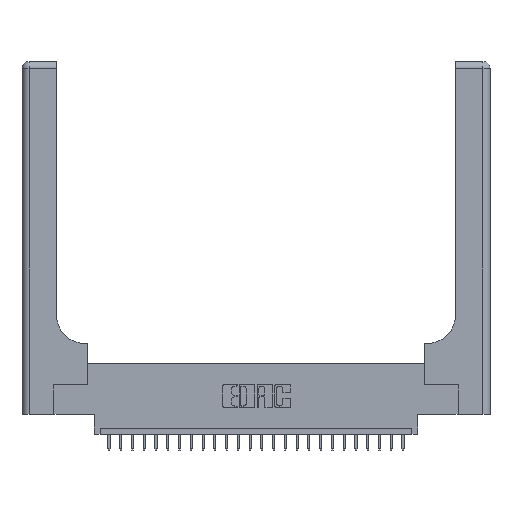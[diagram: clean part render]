
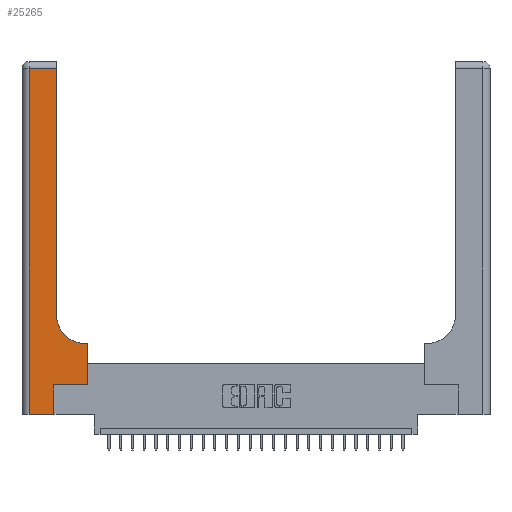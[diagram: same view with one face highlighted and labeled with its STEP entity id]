
A CAD part, top view. The second image highlights one B-rep face of the part: STEP entity #25265.
In plain terms, the highlighted planar face has unit normal (0, 0, 1).
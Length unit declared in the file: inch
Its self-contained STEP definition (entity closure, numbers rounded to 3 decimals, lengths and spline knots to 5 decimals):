
#173 = FACE_OUTER_BOUND ( 'NONE', #19217, .T. ) ;
#336 = EDGE_CURVE ( 'NONE', #24776, #21754, #4469, .T. ) ;
#856 = CARTESIAN_POINT ( 'NONE',  ( 0.2915, 3., 0.37 ) ) ;
#1157 = VERTEX_POINT ( 'NONE', #17591 ) ;
#1690 = VECTOR ( 'NONE', #5617, 39.37008 ) ;
#2215 = PLANE ( 'NONE',  #20758 ) ;
#3052 = VECTOR ( 'NONE', #19072, 39.37008 ) ;
#3142 = DIRECTION ( 'NONE',  ( 1., 0., 0. ) ) ;
#3426 = CIRCLE ( 'NONE', #19691, 0.25 ) ;
#4469 = LINE ( 'NONE', #856, #15046 ) ;
#4856 = CARTESIAN_POINT ( 'NONE',  ( 0.269, 0., 0.37 ) ) ;
#5480 = VECTOR ( 'NONE', #9628, 39.37008 ) ;
#5617 = DIRECTION ( 'NONE',  ( 1., 0., 0. ) ) ;
#5898 = ORIENTED_EDGE ( 'NONE', *, *, #18238, .T. ) ;
#6192 = CARTESIAN_POINT ( 'NONE',  ( 0.269, 0., 0.37 ) ) ;
#6291 = CARTESIAN_POINT ( 'NONE',  ( 0.2915, 2.94, 0.37 ) ) ;
#7305 = LINE ( 'NONE', #24150, #12107 ) ;
#7981 = DIRECTION ( 'NONE',  ( 1., 0., 0. ) ) ;
#8117 = CARTESIAN_POINT ( 'NONE',  ( 0.06, 2.94, 0.37 ) ) ;
#8766 = DIRECTION ( 'NONE',  ( 0., 1., 0. ) ) ;
#9373 = CARTESIAN_POINT ( 'NONE',  ( 0.06, 3., 0.37 ) ) ;
#9628 = DIRECTION ( 'NONE',  ( 0., -1., 0. ) ) ;
#10048 = CARTESIAN_POINT ( 'NONE',  ( 0.5415, 0.85, 0.37 ) ) ;
#10485 = VERTEX_POINT ( 'NONE', #26332 ) ;
#11897 = DIRECTION ( 'NONE',  ( -1., 0., 0. ) ) ;
#12107 = VECTOR ( 'NONE', #3142, 39.37008 ) ;
#12230 = LINE ( 'NONE', #6192, #26948 ) ;
#12709 = ORIENTED_EDGE ( 'NONE', *, *, #25765, .T. ) ;
#12770 = VERTEX_POINT ( 'NONE', #22653 ) ;
#12938 = ORIENTED_EDGE ( 'NONE', *, *, #22684, .T. ) ;
#13217 = VECTOR ( 'NONE', #22682, 39.37008 ) ;
#13233 = CARTESIAN_POINT ( 'NONE',  ( 0.5415, 0.6, 0.37 ) ) ;
#13918 = ORIENTED_EDGE ( 'NONE', *, *, #21764, .T. ) ;
#13954 = CARTESIAN_POINT ( 'NONE',  ( 0.2915, 0.6, 0.37 ) ) ;
#14596 = EDGE_CURVE ( 'NONE', #10485, #17119, #7305, .T. ) ;
#14833 = ORIENTED_EDGE ( 'NONE', *, *, #25785, .T. ) ;
#15046 = VECTOR ( 'NONE', #8766, 39.37008 ) ;
#16049 = LINE ( 'NONE', #24521, #1690 ) ;
#16080 = DIRECTION ( 'NONE',  ( 0., 0., -1. ) ) ;
#16294 = CARTESIAN_POINT ( 'NONE',  ( 0.269, 0.25, 0.37 ) ) ;
#16975 = DIRECTION ( 'NONE',  ( 0., 0., -1. ) ) ;
#17119 = VERTEX_POINT ( 'NONE', #4856 ) ;
#17133 = VERTEX_POINT ( 'NONE', #13233 ) ;
#17591 = CARTESIAN_POINT ( 'NONE',  ( 0.5585, 0.6, 0.37 ) ) ;
#17666 = VERTEX_POINT ( 'NONE', #16294 ) ;
#17807 = LINE ( 'NONE', #13954, #24451 ) ;
#18238 = EDGE_CURVE ( 'NONE', #17133, #24776, #3426, .T. ) ;
#18858 = ORIENTED_EDGE ( 'NONE', *, *, #336, .T. ) ;
#19072 = DIRECTION ( 'NONE',  ( 0., 1., 0. ) ) ;
#19217 = EDGE_LOOP ( 'NONE', ( #18858, #12938, #12709, #26934, #14833, #20153, #13918, #20929, #5898 ) ) ;
#19249 = VERTEX_POINT ( 'NONE', #8117 ) ;
#19691 = AXIS2_PLACEMENT_3D ( 'NONE', #10048, #16080, #7981 ) ;
#20153 = ORIENTED_EDGE ( 'NONE', *, *, #20202, .T. ) ;
#20202 = EDGE_CURVE ( 'NONE', #17666, #12770, #16049, .T. ) ;
#20460 = LINE ( 'NONE', #9373, #5480 ) ;
#20758 = AXIS2_PLACEMENT_3D ( 'NONE', #21221, #16975, #25290 ) ;
#20929 = ORIENTED_EDGE ( 'NONE', *, *, #26459, .T. ) ;
#21221 = CARTESIAN_POINT ( 'NONE',  ( 0., 3., 0.37 ) ) ;
#21754 = VERTEX_POINT ( 'NONE', #6291 ) ;
#21764 = EDGE_CURVE ( 'NONE', #12770, #1157, #25187, .T. ) ;
#22405 = CARTESIAN_POINT ( 'NONE',  ( 0.2915, 0.85, 0.37 ) ) ;
#22653 = CARTESIAN_POINT ( 'NONE',  ( 0.5585, 0.25, 0.37 ) ) ;
#22682 = DIRECTION ( 'NONE',  ( -1., 0., 0. ) ) ;
#22684 = EDGE_CURVE ( 'NONE', #21754, #19249, #24724, .T. ) ;
#22777 = DIRECTION ( 'NONE',  ( 0., 1., 0. ) ) ;
#23145 = CARTESIAN_POINT ( 'NONE',  ( 0.5585, 0.25, 0.37 ) ) ;
#24150 = CARTESIAN_POINT ( 'NONE',  ( 0., 0., 0.37 ) ) ;
#24451 = VECTOR ( 'NONE', #11897, 39.37008 ) ;
#24521 = CARTESIAN_POINT ( 'NONE',  ( 0.269, 0.25, 0.37 ) ) ;
#24724 = LINE ( 'NONE', #26382, #13217 ) ;
#24776 = VERTEX_POINT ( 'NONE', #22405 ) ;
#25187 = LINE ( 'NONE', #23145, #3052 ) ;
#25265 = ADVANCED_FACE ( 'NONE', ( #173 ), #2215, .F. ) ;
#25290 = DIRECTION ( 'NONE',  ( -1., 0., 0. ) ) ;
#25765 = EDGE_CURVE ( 'NONE', #19249, #10485, #20460, .T. ) ;
#25785 = EDGE_CURVE ( 'NONE', #17119, #17666, #12230, .T. ) ;
#26332 = CARTESIAN_POINT ( 'NONE',  ( 0.06, 0., 0.37 ) ) ;
#26382 = CARTESIAN_POINT ( 'NONE',  ( 0., 2.94, 0.37 ) ) ;
#26459 = EDGE_CURVE ( 'NONE', #1157, #17133, #17807, .T. ) ;
#26934 = ORIENTED_EDGE ( 'NONE', *, *, #14596, .T. ) ;
#26948 = VECTOR ( 'NONE', #22777, 39.37008 ) ;
